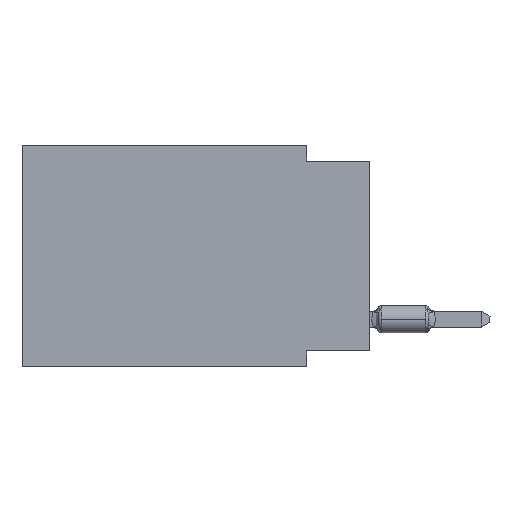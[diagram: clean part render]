
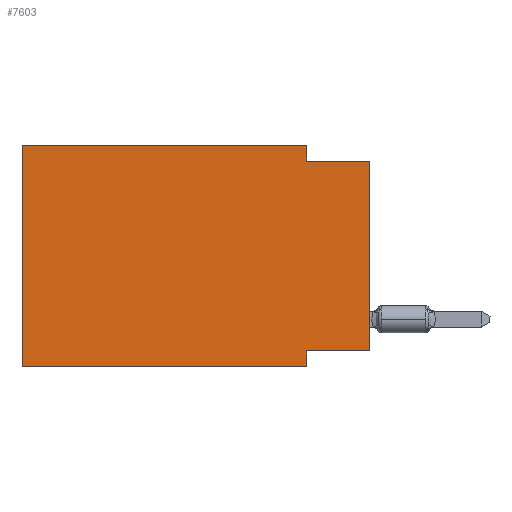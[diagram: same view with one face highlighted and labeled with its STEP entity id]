
A CAD part, left-side view. The second image highlights one B-rep face of the part: STEP entity #7603.
In plain terms, the highlighted planar face has unit normal (-1, 0, 0).
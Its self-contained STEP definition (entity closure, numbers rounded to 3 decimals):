
#2 = EDGE_CURVE ( 'NONE', #10633, #2011, #14244, .T. ) ;
#14 = CARTESIAN_POINT ( 'NONE',  ( 0., 13.97, 0. ) ) ;
#521 = ORIENTED_EDGE ( 'NONE', *, *, #2, .F. ) ;
#704 = VERTEX_POINT ( 'NONE', #9937 ) ;
#990 = DIRECTION ( 'NONE',  ( 1., 0., 0. ) ) ;
#1750 = ORIENTED_EDGE ( 'NONE', *, *, #1901, .F. ) ;
#1901 = EDGE_CURVE ( 'NONE', #2011, #10872, #7293, .T. ) ;
#2011 = VERTEX_POINT ( 'NONE', #14 ) ;
#2118 = CARTESIAN_POINT ( 'NONE',  ( 0., 2.54, -0.635 ) ) ;
#2188 = VECTOR ( 'NONE', #3833, 1000. ) ;
#2211 = ORIENTED_EDGE ( 'NONE', *, *, #5292, .F. ) ;
#2328 = VERTEX_POINT ( 'NONE', #16015 ) ;
#2341 = DIRECTION ( 'NONE',  ( 0., 0., -1. ) ) ;
#2354 = CARTESIAN_POINT ( 'NONE',  ( 0., 2.54, 0. ) ) ;
#2468 = CARTESIAN_POINT ( 'NONE',  ( 0., 0., -8.255 ) ) ;
#2698 = VECTOR ( 'NONE', #2341, 1000. ) ;
#2827 = ORIENTED_EDGE ( 'NONE', *, *, #3453, .T. ) ;
#2950 = CARTESIAN_POINT ( 'NONE',  ( 0., 13.97, -8.89 ) ) ;
#3453 = EDGE_CURVE ( 'NONE', #10633, #2328, #7965, .T. ) ;
#3833 = DIRECTION ( 'NONE',  ( 0., 0., 1. ) ) ;
#4059 = CARTESIAN_POINT ( 'NONE',  ( 0., 13.97, -8.89 ) ) ;
#4776 = LINE ( 'NONE', #15325, #5572 ) ;
#4790 = FACE_OUTER_BOUND ( 'NONE', #15410, .T. ) ;
#5008 = CARTESIAN_POINT ( 'NONE',  ( 0., 2.54, -8.89 ) ) ;
#5161 = VECTOR ( 'NONE', #9709, 1000. ) ;
#5292 = EDGE_CURVE ( 'NONE', #704, #11206, #10249, .T. ) ;
#5328 = ORIENTED_EDGE ( 'NONE', *, *, #14416, .F. ) ;
#5329 = CARTESIAN_POINT ( 'NONE',  ( 0., 2.54, -8.255 ) ) ;
#5447 = VECTOR ( 'NONE', #15469, 1000. ) ;
#5572 = VECTOR ( 'NONE', #11156, 1000. ) ;
#5802 = ORIENTED_EDGE ( 'NONE', *, *, #8386, .F. ) ;
#5951 = ORIENTED_EDGE ( 'NONE', *, *, #14803, .F. ) ;
#6032 = PLANE ( 'NONE',  #13034 ) ;
#6152 = CARTESIAN_POINT ( 'NONE',  ( 0., 2.54, 0. ) ) ;
#6318 = ORIENTED_EDGE ( 'NONE', *, *, #13435, .T. ) ;
#7097 = VERTEX_POINT ( 'NONE', #9382 ) ;
#7293 = LINE ( 'NONE', #8450, #11390 ) ;
#7384 = CARTESIAN_POINT ( 'NONE',  ( 0., 0., -0.635 ) ) ;
#7503 = DIRECTION ( 'NONE',  ( 0., 0., -1. ) ) ;
#7603 = ADVANCED_FACE ( 'NONE', ( #4790 ), #6032, .F. ) ;
#7614 = VECTOR ( 'NONE', #13860, 1000. ) ;
#7965 = LINE ( 'NONE', #4059, #5447 ) ;
#8386 = EDGE_CURVE ( 'NONE', #15444, #7097, #9876, .T. ) ;
#8450 = CARTESIAN_POINT ( 'NONE',  ( 0., 13.97, 0. ) ) ;
#8563 = LINE ( 'NONE', #6152, #2698 ) ;
#8831 = LINE ( 'NONE', #5008, #11930 ) ;
#9382 = CARTESIAN_POINT ( 'NONE',  ( 0., 0., -0.635 ) ) ;
#9709 = DIRECTION ( 'NONE',  ( 0., -1., 0. ) ) ;
#9876 = LINE ( 'NONE', #7384, #5161 ) ;
#9937 = CARTESIAN_POINT ( 'NONE',  ( 0., 0., -8.255 ) ) ;
#10249 = LINE ( 'NONE', #2468, #7614 ) ;
#10633 = VERTEX_POINT ( 'NONE', #2950 ) ;
#10872 = VERTEX_POINT ( 'NONE', #2354 ) ;
#11156 = DIRECTION ( 'NONE',  ( 0., 0., 1. ) ) ;
#11206 = VERTEX_POINT ( 'NONE', #5329 ) ;
#11390 = VECTOR ( 'NONE', #15954, 1000. ) ;
#11930 = VECTOR ( 'NONE', #7503, 1000. ) ;
#12145 = DIRECTION ( 'NONE',  ( 0., 0., -1. ) ) ;
#12313 = CARTESIAN_POINT ( 'NONE',  ( 0., 13.97, 0. ) ) ;
#13034 = AXIS2_PLACEMENT_3D ( 'NONE', #12313, #990, #12145 ) ;
#13435 = EDGE_CURVE ( 'NONE', #704, #7097, #4776, .T. ) ;
#13860 = DIRECTION ( 'NONE',  ( 0., 1., 0. ) ) ;
#13915 = CARTESIAN_POINT ( 'NONE',  ( 0., 13.97, 0. ) ) ;
#14244 = LINE ( 'NONE', #13915, #2188 ) ;
#14416 = EDGE_CURVE ( 'NONE', #11206, #2328, #8831, .T. ) ;
#14803 = EDGE_CURVE ( 'NONE', #10872, #15444, #8563, .T. ) ;
#15325 = CARTESIAN_POINT ( 'NONE',  ( 0., 0., 0. ) ) ;
#15410 = EDGE_LOOP ( 'NONE', ( #6318, #5802, #5951, #1750, #521, #2827, #5328, #2211 ) ) ;
#15444 = VERTEX_POINT ( 'NONE', #2118 ) ;
#15469 = DIRECTION ( 'NONE',  ( 0., -1., 0. ) ) ;
#15954 = DIRECTION ( 'NONE',  ( 0., -1., 0. ) ) ;
#16015 = CARTESIAN_POINT ( 'NONE',  ( 0., 2.54, -8.89 ) ) ;
